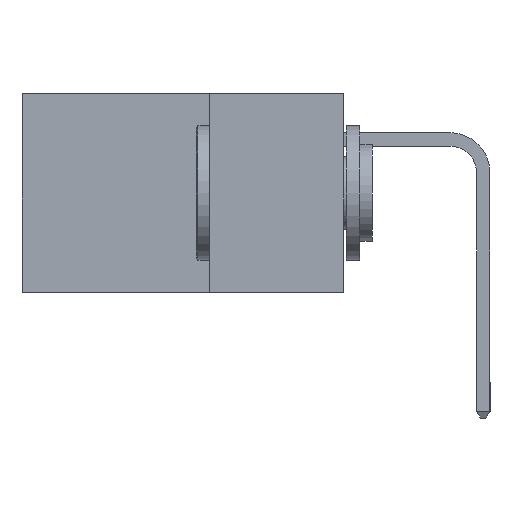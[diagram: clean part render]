
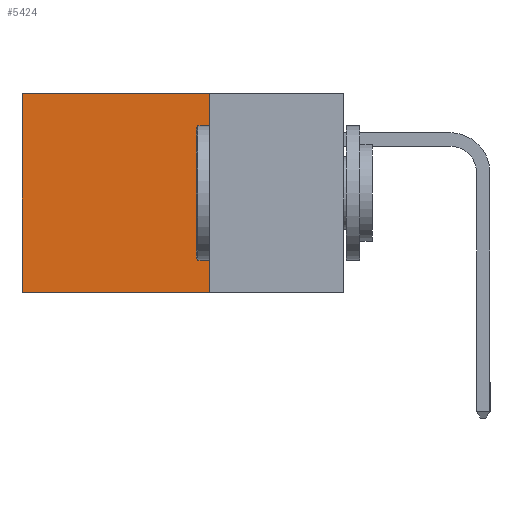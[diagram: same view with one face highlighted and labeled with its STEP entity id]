
A CAD part, left-side view. The second image highlights one B-rep face of the part: STEP entity #5424.
In plain terms, the highlighted planar face has unit normal (-1, 0, 0).
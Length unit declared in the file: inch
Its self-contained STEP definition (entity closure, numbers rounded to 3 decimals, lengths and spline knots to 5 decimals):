
#89 = VECTOR ( 'NONE', #9531, 39.37008 ) ;
#721 = EDGE_CURVE ( 'NONE', #4515, #9898, #8136, .T. ) ;
#1318 = CARTESIAN_POINT ( 'NONE',  ( 0.2615, 0.25, 0. ) ) ;
#2241 = LINE ( 'NONE', #4444, #6201 ) ;
#3397 = VECTOR ( 'NONE', #10030, 39.37008 ) ;
#3473 = EDGE_LOOP ( 'NONE', ( #12055, #9822, #11500, #10984 ) ) ;
#3588 = EDGE_CURVE ( 'NONE', #8604, #9898, #3706, .T. ) ;
#3706 = LINE ( 'NONE', #6764, #89 ) ;
#3802 = CARTESIAN_POINT ( 'NONE',  ( 0.2615, 0.6, -0.37 ) ) ;
#4444 = CARTESIAN_POINT ( 'NONE',  ( 0.2615, 0.25, -0.37 ) ) ;
#4515 = VERTEX_POINT ( 'NONE', #10592 ) ;
#5424 = ADVANCED_FACE ( 'NONE', ( #11971 ), #7860, .F. ) ;
#5445 = LINE ( 'NONE', #1318, #12248 ) ;
#6013 = CARTESIAN_POINT ( 'NONE',  ( 0.2615, 0.25, 0. ) ) ;
#6040 = CARTESIAN_POINT ( 'NONE',  ( 0.2615, 0.6, -0.37 ) ) ;
#6088 = CARTESIAN_POINT ( 'NONE',  ( 0.2615, 0.25, -0.37 ) ) ;
#6201 = VECTOR ( 'NONE', #12105, 39.37008 ) ;
#6764 = CARTESIAN_POINT ( 'NONE',  ( 0.2615, 0.25, -0.37 ) ) ;
#7860 = PLANE ( 'NONE',  #10138 ) ;
#8136 = LINE ( 'NONE', #6040, #3397 ) ;
#8604 = VERTEX_POINT ( 'NONE', #11391 ) ;
#9531 = DIRECTION ( 'NONE',  ( 0., 1., 0. ) ) ;
#9822 = ORIENTED_EDGE ( 'NONE', *, *, #3588, .F. ) ;
#9898 = VERTEX_POINT ( 'NONE', #3802 ) ;
#10030 = DIRECTION ( 'NONE',  ( 0., 0., -1. ) ) ;
#10138 = AXIS2_PLACEMENT_3D ( 'NONE', #6088, #11847, #12890 ) ;
#10592 = CARTESIAN_POINT ( 'NONE',  ( 0.2615, 0.6, 0. ) ) ;
#10984 = ORIENTED_EDGE ( 'NONE', *, *, #11018, .T. ) ;
#11018 = EDGE_CURVE ( 'NONE', #11887, #4515, #5445, .T. ) ;
#11391 = CARTESIAN_POINT ( 'NONE',  ( 0.2615, 0.25, -0.37 ) ) ;
#11464 = DIRECTION ( 'NONE',  ( 0., 1., 0. ) ) ;
#11497 = EDGE_CURVE ( 'NONE', #11887, #8604, #2241, .T. ) ;
#11500 = ORIENTED_EDGE ( 'NONE', *, *, #11497, .F. ) ;
#11847 = DIRECTION ( 'NONE',  ( 1., 0., 0. ) ) ;
#11887 = VERTEX_POINT ( 'NONE', #6013 ) ;
#11971 = FACE_OUTER_BOUND ( 'NONE', #3473, .T. ) ;
#12055 = ORIENTED_EDGE ( 'NONE', *, *, #721, .T. ) ;
#12105 = DIRECTION ( 'NONE',  ( 0., 0., -1. ) ) ;
#12248 = VECTOR ( 'NONE', #11464, 39.37008 ) ;
#12890 = DIRECTION ( 'NONE',  ( 0., 0., -1. ) ) ;
